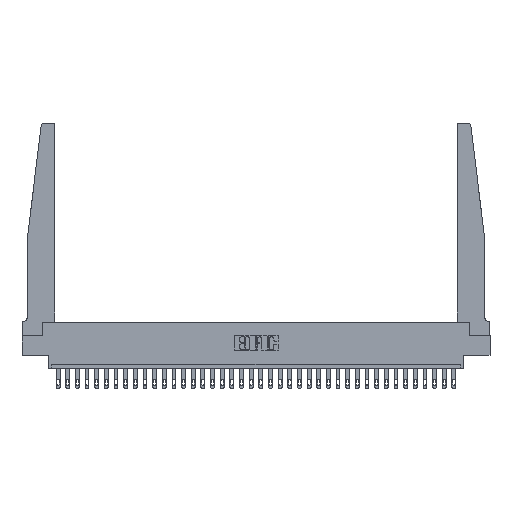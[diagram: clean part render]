
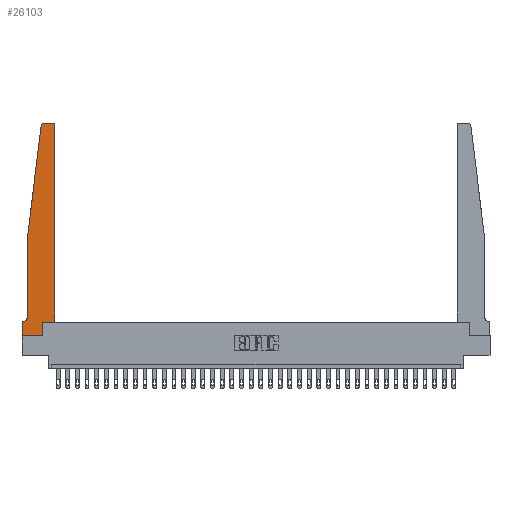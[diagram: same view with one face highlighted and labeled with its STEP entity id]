
A CAD part, top view. The second image highlights one B-rep face of the part: STEP entity #26103.
In plain terms, the highlighted planar face has unit normal (0, 0, 1).
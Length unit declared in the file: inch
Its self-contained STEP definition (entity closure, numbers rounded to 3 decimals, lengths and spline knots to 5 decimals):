
#199 = CARTESIAN_POINT ( 'NONE',  ( 0.015, 0.1875, 0.37 ) ) ;
#260 = DIRECTION ( 'NONE',  ( 0., 0., 1. ) ) ;
#915 = DIRECTION ( 'NONE',  ( 0., 1., 0. ) ) ;
#1060 = ORIENTED_EDGE ( 'NONE', *, *, #30154, .T. ) ;
#1210 = ORIENTED_EDGE ( 'NONE', *, *, #25591, .T. ) ;
#1270 = DIRECTION ( 'NONE',  ( -1., 0., 0. ) ) ;
#1271 = CARTESIAN_POINT ( 'NONE',  ( 0.065, 1.25, 0.37 ) ) ;
#1793 = DIRECTION ( 'NONE',  ( -1., 0., 0. ) ) ;
#1933 = VECTOR ( 'NONE', #4422, 39.37008 ) ;
#2695 = CIRCLE ( 'NONE', #20436, 0.03 ) ;
#3146 = CARTESIAN_POINT ( 'NONE',  ( 0.2605, 0.18, 0.37 ) ) ;
#3183 = CARTESIAN_POINT ( 'NONE',  ( 0., 0., 0.37 ) ) ;
#3662 = LINE ( 'NONE', #13339, #17182 ) ;
#3728 = VERTEX_POINT ( 'NONE', #199 ) ;
#4006 = VECTOR ( 'NONE', #26608, 39.37008 ) ;
#4422 = DIRECTION ( 'NONE',  ( 0., -1., 0. ) ) ;
#4460 = LINE ( 'NONE', #16663, #24631 ) ;
#4918 = AXIS2_PLACEMENT_3D ( 'NONE', #24856, #260, #7584 ) ;
#5171 = ORIENTED_EDGE ( 'NONE', *, *, #28404, .T. ) ;
#5773 = ORIENTED_EDGE ( 'NONE', *, *, #12608, .T. ) ;
#6791 = CARTESIAN_POINT ( 'NONE',  ( 0.27653, 2.72, 0.37 ) ) ;
#6956 = DIRECTION ( 'NONE',  ( 0., 0., 1. ) ) ;
#7320 = DIRECTION ( 'NONE',  ( 1., 0., 0. ) ) ;
#7584 = DIRECTION ( 'NONE',  ( 1., 0., 0. ) ) ;
#7746 = CARTESIAN_POINT ( 'NONE',  ( 0.24675, 2.72367, 0.37 ) ) ;
#8011 = VECTOR ( 'NONE', #19784, 39.37008 ) ;
#8283 = CARTESIAN_POINT ( 'NONE',  ( 0.395, 2.75, 0.37 ) ) ;
#8578 = ORIENTED_EDGE ( 'NONE', *, *, #23346, .T. ) ;
#8976 = VERTEX_POINT ( 'NONE', #7746 ) ;
#9116 = CIRCLE ( 'NONE', #27840, 0.05 ) ;
#9838 = VERTEX_POINT ( 'NONE', #3183 ) ;
#10241 = CARTESIAN_POINT ( 'NONE',  ( 0.425, 0.18, 0.37 ) ) ;
#10633 = CARTESIAN_POINT ( 'NONE',  ( 0.27653, 2.75, 0.37 ) ) ;
#11520 = ORIENTED_EDGE ( 'NONE', *, *, #19223, .T. ) ;
#12142 = DIRECTION ( 'NONE',  ( 1., 0., 0. ) ) ;
#12438 = ORIENTED_EDGE ( 'NONE', *, *, #13459, .T. ) ;
#12593 = VECTOR ( 'NONE', #12142, 39.37008 ) ;
#12608 = EDGE_CURVE ( 'NONE', #9838, #17113, #24287, .T. ) ;
#13058 = DIRECTION ( 'NONE',  ( 0., -1., 0. ) ) ;
#13231 = VERTEX_POINT ( 'NONE', #1271 ) ;
#13339 = CARTESIAN_POINT ( 'NONE',  ( 0.25, 2.75, 0.37 ) ) ;
#13459 = EDGE_CURVE ( 'NONE', #25000, #26602, #2695, .T. ) ;
#13557 = DIRECTION ( 'NONE',  ( 0., 0., -1. ) ) ;
#14130 = DIRECTION ( 'NONE',  ( 0., 0., 1. ) ) ;
#14285 = DIRECTION ( 'NONE',  ( 1., 0., 0. ) ) ;
#14805 = ORIENTED_EDGE ( 'NONE', *, *, #27862, .T. ) ;
#14824 = CARTESIAN_POINT ( 'NONE',  ( 0.2605, 0., 0.37 ) ) ;
#15025 = CARTESIAN_POINT ( 'NONE',  ( 0.065, 0.1875, 0.37 ) ) ;
#15280 = VERTEX_POINT ( 'NONE', #24703 ) ;
#16629 = LINE ( 'NONE', #18853, #1933 ) ;
#16663 = CARTESIAN_POINT ( 'NONE',  ( 0.065, 1.25, 0.37 ) ) ;
#16928 = DIRECTION ( 'NONE',  ( 1., 0., 0. ) ) ;
#17086 = VERTEX_POINT ( 'NONE', #22289 ) ;
#17113 = VERTEX_POINT ( 'NONE', #14824 ) ;
#17182 = VECTOR ( 'NONE', #1270, 39.37008 ) ;
#17923 = VECTOR ( 'NONE', #7320, 39.37008 ) ;
#18087 = ORIENTED_EDGE ( 'NONE', *, *, #28477, .T. ) ;
#18853 = CARTESIAN_POINT ( 'NONE',  ( 0.065, 1.25, 0.37 ) ) ;
#19223 = EDGE_CURVE ( 'NONE', #8976, #13231, #4460, .T. ) ;
#19784 = DIRECTION ( 'NONE',  ( -1., 0., 0. ) ) ;
#19922 = VECTOR ( 'NONE', #13058, 39.37008 ) ;
#19932 = FACE_OUTER_BOUND ( 'NONE', #26618, .T. ) ;
#20057 = CARTESIAN_POINT ( 'NONE',  ( 0.425, 2.72, 0.37 ) ) ;
#20436 = AXIS2_PLACEMENT_3D ( 'NONE', #23463, #14130, #14285 ) ;
#21009 = CARTESIAN_POINT ( 'NONE',  ( 0.015, 0.2375, 0.37 ) ) ;
#21220 = VERTEX_POINT ( 'NONE', #27151 ) ;
#21709 = CARTESIAN_POINT ( 'NONE',  ( 0.425, 0.18, 0.37 ) ) ;
#21911 = CARTESIAN_POINT ( 'NONE',  ( 0., 0., 0.37 ) ) ;
#22004 = PLANE ( 'NONE',  #4918 ) ;
#22289 = CARTESIAN_POINT ( 'NONE',  ( 0., 0.1875, 0.37 ) ) ;
#22488 = LINE ( 'NONE', #15025, #8011 ) ;
#22537 = EDGE_CURVE ( 'NONE', #17086, #9838, #25091, .T. ) ;
#22647 = LINE ( 'NONE', #3146, #23667 ) ;
#22957 = VERTEX_POINT ( 'NONE', #10633 ) ;
#23346 = EDGE_CURVE ( 'NONE', #17113, #15280, #22647, .T. ) ;
#23463 = CARTESIAN_POINT ( 'NONE',  ( 0.395, 2.72, 0.37 ) ) ;
#23667 = VECTOR ( 'NONE', #915, 39.37008 ) ;
#24287 = LINE ( 'NONE', #21911, #17923 ) ;
#24341 = EDGE_CURVE ( 'NONE', #13231, #29487, #16629, .T. ) ;
#24631 = VECTOR ( 'NONE', #28854, 39.37008 ) ;
#24703 = CARTESIAN_POINT ( 'NONE',  ( 0.2605, 0.18, 0.37 ) ) ;
#24856 = CARTESIAN_POINT ( 'NONE',  ( 0., 0.1875, 0.37 ) ) ;
#25000 = VERTEX_POINT ( 'NONE', #20057 ) ;
#25091 = LINE ( 'NONE', #25249, #19922 ) ;
#25249 = CARTESIAN_POINT ( 'NONE',  ( 0., 0., 0.37 ) ) ;
#25264 = AXIS2_PLACEMENT_3D ( 'NONE', #6791, #6956, #16928 ) ;
#25271 = ORIENTED_EDGE ( 'NONE', *, *, #27389, .T. ) ;
#25591 = EDGE_CURVE ( 'NONE', #26602, #22957, #3662, .T. ) ;
#26103 = ADVANCED_FACE ( 'NONE', ( #19932 ), #22004, .T. ) ;
#26602 = VERTEX_POINT ( 'NONE', #8283 ) ;
#26608 = DIRECTION ( 'NONE',  ( 0., 1., 0. ) ) ;
#26618 = EDGE_LOOP ( 'NONE', ( #1210, #5171, #11520, #26767, #1060, #25271, #29374, #5773, #8578, #14805, #18087, #12438 ) ) ;
#26767 = ORIENTED_EDGE ( 'NONE', *, *, #24341, .T. ) ;
#27151 = CARTESIAN_POINT ( 'NONE',  ( 0.425, 0.18, 0.37 ) ) ;
#27389 = EDGE_CURVE ( 'NONE', #3728, #17086, #22488, .T. ) ;
#27840 = AXIS2_PLACEMENT_3D ( 'NONE', #21009, #13557, #1793 ) ;
#27862 = EDGE_CURVE ( 'NONE', #15280, #21220, #29716, .T. ) ;
#28404 = EDGE_CURVE ( 'NONE', #22957, #8976, #29294, .T. ) ;
#28477 = EDGE_CURVE ( 'NONE', #21220, #25000, #28502, .T. ) ;
#28502 = LINE ( 'NONE', #21709, #4006 ) ;
#28854 = DIRECTION ( 'NONE',  ( -0.122, -0.992, 0. ) ) ;
#29294 = CIRCLE ( 'NONE', #25264, 0.03 ) ;
#29374 = ORIENTED_EDGE ( 'NONE', *, *, #22537, .T. ) ;
#29487 = VERTEX_POINT ( 'NONE', #31241 ) ;
#29716 = LINE ( 'NONE', #10241, #12593 ) ;
#30154 = EDGE_CURVE ( 'NONE', #29487, #3728, #9116, .T. ) ;
#31241 = CARTESIAN_POINT ( 'NONE',  ( 0.065, 0.2375, 0.37 ) ) ;
